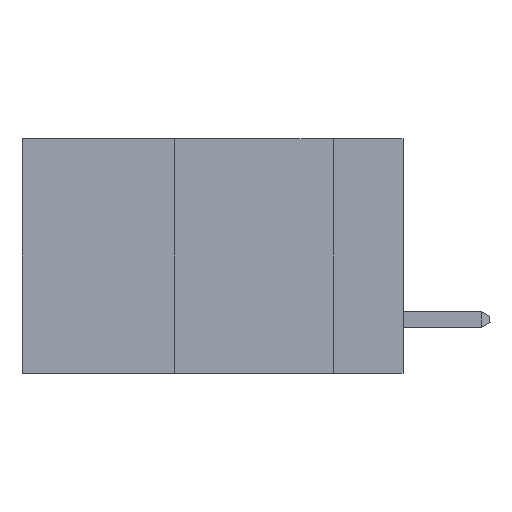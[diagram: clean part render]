
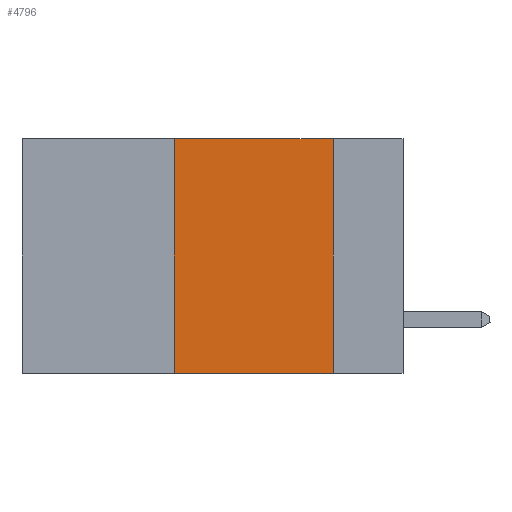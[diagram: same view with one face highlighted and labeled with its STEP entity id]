
A CAD part, left-side view. The second image highlights one B-rep face of the part: STEP entity #4796.
In plain terms, the highlighted planar face has unit normal (-1, 0, 0).
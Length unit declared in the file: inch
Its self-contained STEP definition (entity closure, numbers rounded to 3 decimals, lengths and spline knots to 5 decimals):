
#257 = EDGE_CURVE ( 'NONE', #11118, #23974, #8459, .T. ) ;
#1722 = CARTESIAN_POINT ( 'NONE',  ( 0., 0.11, 0. ) ) ;
#2611 = DIRECTION ( 'NONE',  ( 0., 0., -1. ) ) ;
#2820 = LINE ( 'NONE', #12372, #9793 ) ;
#4103 = AXIS2_PLACEMENT_3D ( 'NONE', #9286, #11437, #2611 ) ;
#4251 = ORIENTED_EDGE ( 'NONE', *, *, #23405, .F. ) ;
#4796 = ADVANCED_FACE ( 'NONE', ( #17220 ), #19719, .F. ) ;
#5003 = EDGE_CURVE ( 'NONE', #9456, #23974, #8615, .T. ) ;
#6033 = DIRECTION ( 'NONE',  ( 0., 0., 1. ) ) ;
#6541 = ORIENTED_EDGE ( 'NONE', *, *, #257, .T. ) ;
#7120 = VECTOR ( 'NONE', #11008, 39.37008 ) ;
#8229 = CARTESIAN_POINT ( 'NONE',  ( 0., 0.11, -0.37 ) ) ;
#8459 = LINE ( 'NONE', #27297, #7120 ) ;
#8615 = LINE ( 'NONE', #1722, #23531 ) ;
#9286 = CARTESIAN_POINT ( 'NONE',  ( 0., 0.6, 0. ) ) ;
#9456 = VERTEX_POINT ( 'NONE', #23016 ) ;
#9793 = VECTOR ( 'NONE', #6033, 39.37008 ) ;
#11008 = DIRECTION ( 'NONE',  ( 0., -1., 0. ) ) ;
#11031 = VERTEX_POINT ( 'NONE', #13758 ) ;
#11118 = VERTEX_POINT ( 'NONE', #14297 ) ;
#11437 = DIRECTION ( 'NONE',  ( 1., 0., 0. ) ) ;
#12022 = ORIENTED_EDGE ( 'NONE', *, *, #24463, .F. ) ;
#12070 = LINE ( 'NONE', #14156, #14762 ) ;
#12372 = CARTESIAN_POINT ( 'NONE',  ( 0., 0.36, 0. ) ) ;
#13758 = CARTESIAN_POINT ( 'NONE',  ( 0., 0.36, 0. ) ) ;
#14156 = CARTESIAN_POINT ( 'NONE',  ( 0., 0.6, 0. ) ) ;
#14297 = CARTESIAN_POINT ( 'NONE',  ( 0., 0.36, -0.37 ) ) ;
#14762 = VECTOR ( 'NONE', #18191, 39.37008 ) ;
#14841 = DIRECTION ( 'NONE',  ( 0., 0., -1. ) ) ;
#17220 = FACE_OUTER_BOUND ( 'NONE', #24047, .T. ) ;
#18191 = DIRECTION ( 'NONE',  ( 0., -1., 0. ) ) ;
#19162 = ORIENTED_EDGE ( 'NONE', *, *, #5003, .F. ) ;
#19719 = PLANE ( 'NONE',  #4103 ) ;
#23016 = CARTESIAN_POINT ( 'NONE',  ( 0., 0.11, 0. ) ) ;
#23405 = EDGE_CURVE ( 'NONE', #11118, #11031, #2820, .T. ) ;
#23531 = VECTOR ( 'NONE', #14841, 39.37008 ) ;
#23974 = VERTEX_POINT ( 'NONE', #8229 ) ;
#24047 = EDGE_LOOP ( 'NONE', ( #19162, #12022, #4251, #6541 ) ) ;
#24463 = EDGE_CURVE ( 'NONE', #11031, #9456, #12070, .T. ) ;
#27297 = CARTESIAN_POINT ( 'NONE',  ( 0., 0.6, -0.37 ) ) ;
